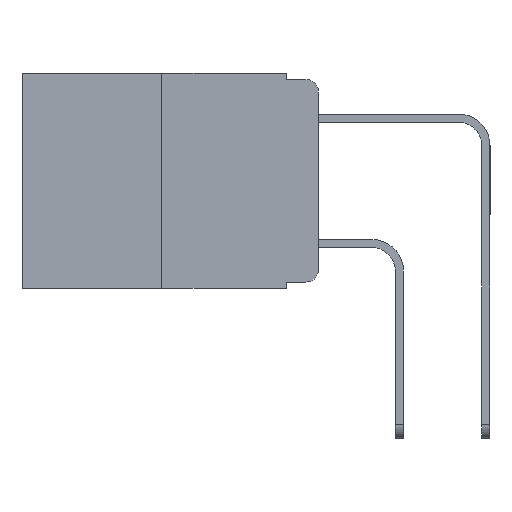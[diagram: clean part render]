
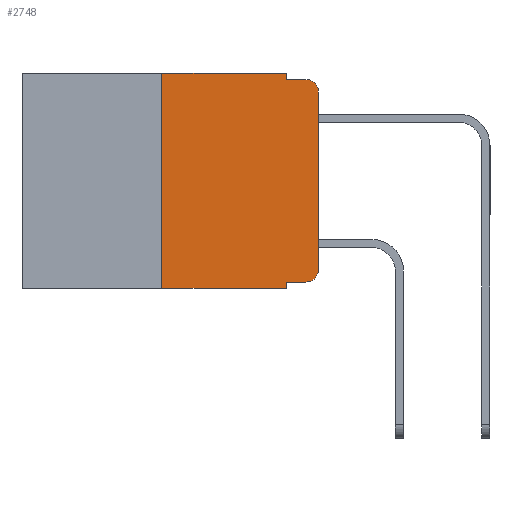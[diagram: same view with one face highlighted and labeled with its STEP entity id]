
A CAD part, left-side view. The second image highlights one B-rep face of the part: STEP entity #2748.
In plain terms, the highlighted planar face has unit normal (-1, 0, 0).
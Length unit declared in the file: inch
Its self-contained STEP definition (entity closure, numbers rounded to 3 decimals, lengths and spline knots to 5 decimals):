
#24 = LINE ( 'NONE', #8949, #8725 ) ;
#577 = CARTESIAN_POINT ( 'NONE',  ( 0., 0.473, -0.343 ) ) ;
#1064 = CARTESIAN_POINT ( 'NONE',  ( 0., 0., -0.03 ) ) ;
#1314 = LINE ( 'NONE', #577, #18658 ) ;
#1433 = CARTESIAN_POINT ( 'NONE',  ( 0., 0.02, -0.03 ) ) ;
#1568 = CARTESIAN_POINT ( 'NONE',  ( 0., 0.473, 0. ) ) ;
#1651 = LINE ( 'NONE', #3914, #10293 ) ;
#2342 = EDGE_CURVE ( 'NONE', #7863, #4362, #20446, .T. ) ;
#2709 = CARTESIAN_POINT ( 'NONE',  ( 0., 0.25, 0. ) ) ;
#2748 = ADVANCED_FACE ( 'NONE', ( #15162 ), #16469, .F. ) ;
#2830 = VERTEX_POINT ( 'NONE', #3433 ) ;
#3178 = DIRECTION ( 'NONE',  ( 0., 0., -1. ) ) ;
#3275 = VECTOR ( 'NONE', #15152, 39.37008 ) ;
#3433 = CARTESIAN_POINT ( 'NONE',  ( 0., 0.02, -0.333 ) ) ;
#3914 = CARTESIAN_POINT ( 'NONE',  ( 0., 0.051, -0.01 ) ) ;
#3964 = DIRECTION ( 'NONE',  ( -1., 0., 0. ) ) ;
#4362 = VERTEX_POINT ( 'NONE', #16831 ) ;
#5254 = LINE ( 'NONE', #2709, #9806 ) ;
#5321 = VERTEX_POINT ( 'NONE', #13432 ) ;
#5360 = ORIENTED_EDGE ( 'NONE', *, *, #11004, .T. ) ;
#5501 = CARTESIAN_POINT ( 'NONE',  ( 0., 0.25, -0.343 ) ) ;
#5599 = CARTESIAN_POINT ( 'NONE',  ( 0., 0.051, -0.333 ) ) ;
#5856 = EDGE_LOOP ( 'NONE', ( #8098, #17342, #14590, #10715, #19376, #7263, #20337, #8877, #5360, #10440 ) ) ;
#6251 = DIRECTION ( 'NONE',  ( 0., 0., 1. ) ) ;
#6730 = AXIS2_PLACEMENT_3D ( 'NONE', #14120, #3964, #15736 ) ;
#6756 = EDGE_CURVE ( 'NONE', #11675, #18288, #1314, .T. ) ;
#7263 = ORIENTED_EDGE ( 'NONE', *, *, #14315, .F. ) ;
#7306 = DIRECTION ( 'NONE',  ( 0., 0., -1. ) ) ;
#7591 = VECTOR ( 'NONE', #14009, 39.37008 ) ;
#7863 = VERTEX_POINT ( 'NONE', #8358 ) ;
#8098 = ORIENTED_EDGE ( 'NONE', *, *, #20760, .T. ) ;
#8358 = CARTESIAN_POINT ( 'NONE',  ( 0., 0.25, 0. ) ) ;
#8607 = DIRECTION ( 'NONE',  ( 0., 0., -1. ) ) ;
#8725 = VECTOR ( 'NONE', #7306, 39.37008 ) ;
#8745 = EDGE_CURVE ( 'NONE', #2830, #5321, #15761, .T. ) ;
#8796 = VERTEX_POINT ( 'NONE', #17429 ) ;
#8877 = ORIENTED_EDGE ( 'NONE', *, *, #13234, .F. ) ;
#8949 = CARTESIAN_POINT ( 'NONE',  ( 0., 0.051, 0. ) ) ;
#8953 = CARTESIAN_POINT ( 'NONE',  ( 0., 0.051, -0.343 ) ) ;
#9315 = CARTESIAN_POINT ( 'NONE',  ( 0., 0.02, -0.01 ) ) ;
#9806 = VECTOR ( 'NONE', #6251, 39.37008 ) ;
#10293 = VECTOR ( 'NONE', #20516, 39.37008 ) ;
#10440 = ORIENTED_EDGE ( 'NONE', *, *, #8745, .T. ) ;
#10715 = ORIENTED_EDGE ( 'NONE', *, *, #15391, .F. ) ;
#11004 = EDGE_CURVE ( 'NONE', #8796, #2830, #16386, .T. ) ;
#11542 = AXIS2_PLACEMENT_3D ( 'NONE', #1433, #13412, #3178 ) ;
#11675 = VERTEX_POINT ( 'NONE', #5501 ) ;
#11879 = LINE ( 'NONE', #18337, #14160 ) ;
#13234 = EDGE_CURVE ( 'NONE', #8796, #18288, #15270, .T. ) ;
#13412 = DIRECTION ( 'NONE',  ( -1., 0., 0. ) ) ;
#13432 = CARTESIAN_POINT ( 'NONE',  ( 0., 0., -0.313 ) ) ;
#13556 = DIRECTION ( 'NONE',  ( 0., 0., 1. ) ) ;
#14009 = DIRECTION ( 'NONE',  ( 0., -1., 0. ) ) ;
#14120 = CARTESIAN_POINT ( 'NONE',  ( 0., 0.02, -0.313 ) ) ;
#14160 = VECTOR ( 'NONE', #13556, 39.37008 ) ;
#14315 = EDGE_CURVE ( 'NONE', #11675, #7863, #5254, .T. ) ;
#14349 = VERTEX_POINT ( 'NONE', #1064 ) ;
#14590 = ORIENTED_EDGE ( 'NONE', *, *, #17544, .F. ) ;
#14848 = AXIS2_PLACEMENT_3D ( 'NONE', #18078, #14856, #19694 ) ;
#14856 = DIRECTION ( 'NONE',  ( 1., 0., 0. ) ) ;
#15112 = CIRCLE ( 'NONE', #11542, 0.02 ) ;
#15152 = DIRECTION ( 'NONE',  ( 0., -1., 0. ) ) ;
#15162 = FACE_OUTER_BOUND ( 'NONE', #5856, .T. ) ;
#15270 = LINE ( 'NONE', #18429, #19064 ) ;
#15391 = EDGE_CURVE ( 'NONE', #4362, #18818, #24, .T. ) ;
#15517 = VERTEX_POINT ( 'NONE', #9315 ) ;
#15736 = DIRECTION ( 'NONE',  ( 0., 0., -1. ) ) ;
#15761 = CIRCLE ( 'NONE', #6730, 0.02 ) ;
#15820 = DIRECTION ( 'NONE',  ( 0., -1., 0. ) ) ;
#16386 = LINE ( 'NONE', #5599, #7591 ) ;
#16469 = PLANE ( 'NONE',  #14848 ) ;
#16831 = CARTESIAN_POINT ( 'NONE',  ( 0., 0.051, 0. ) ) ;
#17342 = ORIENTED_EDGE ( 'NONE', *, *, #19695, .T. ) ;
#17429 = CARTESIAN_POINT ( 'NONE',  ( 0., 0.051, -0.333 ) ) ;
#17544 = EDGE_CURVE ( 'NONE', #18818, #15517, #1651, .T. ) ;
#18075 = CARTESIAN_POINT ( 'NONE',  ( 0., 0.051, -0.01 ) ) ;
#18078 = CARTESIAN_POINT ( 'NONE',  ( 0., 0.473, 0. ) ) ;
#18288 = VERTEX_POINT ( 'NONE', #8953 ) ;
#18337 = CARTESIAN_POINT ( 'NONE',  ( 0., 0., 0. ) ) ;
#18429 = CARTESIAN_POINT ( 'NONE',  ( 0., 0.051, 0. ) ) ;
#18658 = VECTOR ( 'NONE', #15820, 39.37008 ) ;
#18818 = VERTEX_POINT ( 'NONE', #18075 ) ;
#19064 = VECTOR ( 'NONE', #8607, 39.37008 ) ;
#19376 = ORIENTED_EDGE ( 'NONE', *, *, #2342, .F. ) ;
#19694 = DIRECTION ( 'NONE',  ( 0., 0., -1. ) ) ;
#19695 = EDGE_CURVE ( 'NONE', #14349, #15517, #15112, .T. ) ;
#20337 = ORIENTED_EDGE ( 'NONE', *, *, #6756, .T. ) ;
#20446 = LINE ( 'NONE', #1568, #3275 ) ;
#20516 = DIRECTION ( 'NONE',  ( 0., -1., 0. ) ) ;
#20760 = EDGE_CURVE ( 'NONE', #5321, #14349, #11879, .T. ) ;
